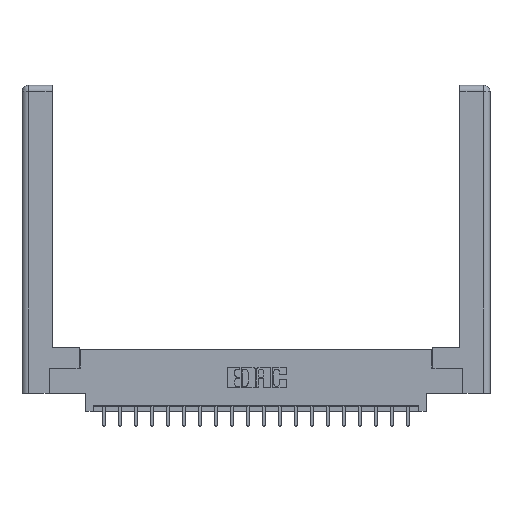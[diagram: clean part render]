
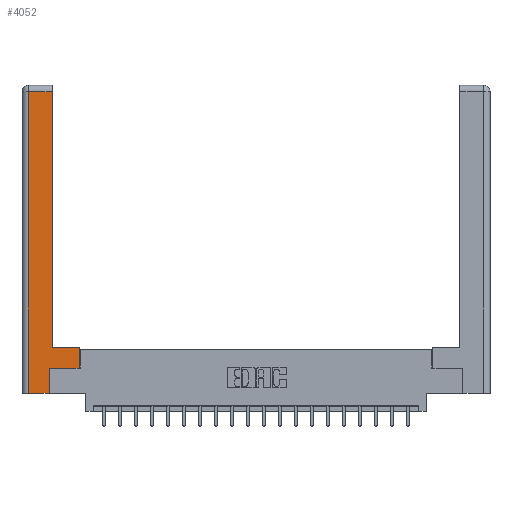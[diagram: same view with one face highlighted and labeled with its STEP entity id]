
A CAD part, top view. The second image highlights one B-rep face of the part: STEP entity #4052.
In plain terms, the highlighted planar face has unit normal (0, 0, 1).
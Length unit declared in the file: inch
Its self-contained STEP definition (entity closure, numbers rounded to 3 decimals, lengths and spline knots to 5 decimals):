
#280 = CARTESIAN_POINT ( 'NONE',  ( 0.0615, 2.94, 0. ) ) ;
#493 = DIRECTION ( 'NONE',  ( 0., 1., 0. ) ) ;
#670 = VECTOR ( 'NONE', #4784, 39.37008 ) ;
#1432 = LINE ( 'NONE', #21107, #670 ) ;
#3005 = ORIENTED_EDGE ( 'NONE', *, *, #5971, .T. ) ;
#3020 = EDGE_LOOP ( 'NONE', ( #16527, #5303, #6921, #6125, #13822, #3005, #13049, #17328 ) ) ;
#3183 = CARTESIAN_POINT ( 'NONE',  ( 0., 0., 0. ) ) ;
#4052 = ADVANCED_FACE ( 'NONE', ( #15620 ), #19458, .F. ) ;
#4313 = VERTEX_POINT ( 'NONE', #19497 ) ;
#4544 = CARTESIAN_POINT ( 'NONE',  ( 0.0615, 2.94, 0. ) ) ;
#4565 = LINE ( 'NONE', #11743, #13985 ) ;
#4569 = VERTEX_POINT ( 'NONE', #10533 ) ;
#4713 = CARTESIAN_POINT ( 'NONE',  ( 0.565, 0.245, 0. ) ) ;
#4784 = DIRECTION ( 'NONE',  ( 0., -1., 0. ) ) ;
#5303 = ORIENTED_EDGE ( 'NONE', *, *, #8015, .T. ) ;
#5707 = EDGE_CURVE ( 'NONE', #9108, #13823, #11936, .T. ) ;
#5791 = DIRECTION ( 'NONE',  ( 0., 0., -1. ) ) ;
#5861 = DIRECTION ( 'NONE',  ( -1., 0., 0. ) ) ;
#5921 = LINE ( 'NONE', #16191, #7468 ) ;
#5971 = EDGE_CURVE ( 'NONE', #13823, #10872, #4565, .T. ) ;
#6061 = CARTESIAN_POINT ( 'NONE',  ( 0.265, 0.245, 0. ) ) ;
#6125 = ORIENTED_EDGE ( 'NONE', *, *, #9671, .T. ) ;
#6391 = DIRECTION ( 'NONE',  ( 0., 1., 0. ) ) ;
#6852 = VECTOR ( 'NONE', #7717, 39.37008 ) ;
#6921 = ORIENTED_EDGE ( 'NONE', *, *, #10904, .T. ) ;
#7195 = CARTESIAN_POINT ( 'NONE',  ( 0.265, 0., 0. ) ) ;
#7468 = VECTOR ( 'NONE', #6391, 39.37008 ) ;
#7717 = DIRECTION ( 'NONE',  ( 1., 0., 0. ) ) ;
#8015 = EDGE_CURVE ( 'NONE', #4569, #14010, #19679, .T. ) ;
#9108 = VERTEX_POINT ( 'NONE', #7195 ) ;
#9671 = EDGE_CURVE ( 'NONE', #19470, #9108, #20620, .T. ) ;
#10533 = CARTESIAN_POINT ( 'NONE',  ( 0.295, 2.94, 0. ) ) ;
#10726 = EDGE_CURVE ( 'NONE', #10872, #4313, #17302, .T. ) ;
#10872 = VERTEX_POINT ( 'NONE', #4713 ) ;
#10904 = EDGE_CURVE ( 'NONE', #14010, #19470, #1432, .T. ) ;
#11191 = AXIS2_PLACEMENT_3D ( 'NONE', #3183, #5791, #5861 ) ;
#11202 = EDGE_CURVE ( 'NONE', #4313, #19335, #16265, .T. ) ;
#11743 = CARTESIAN_POINT ( 'NONE',  ( 0.565, 0.245, 0. ) ) ;
#11847 = CARTESIAN_POINT ( 'NONE',  ( 0.565, 0.45, 0. ) ) ;
#11936 = LINE ( 'NONE', #13193, #20637 ) ;
#11952 = DIRECTION ( 'NONE',  ( 1., 0., 0. ) ) ;
#12536 = VECTOR ( 'NONE', #16879, 39.37008 ) ;
#12959 = VECTOR ( 'NONE', #493, 39.37008 ) ;
#13049 = ORIENTED_EDGE ( 'NONE', *, *, #10726, .T. ) ;
#13193 = CARTESIAN_POINT ( 'NONE',  ( 0.265, 0.245, 0. ) ) ;
#13339 = DIRECTION ( 'NONE',  ( 0., 1., 0. ) ) ;
#13484 = CARTESIAN_POINT ( 'NONE',  ( 0.0615, 0., 0. ) ) ;
#13822 = ORIENTED_EDGE ( 'NONE', *, *, #5707, .T. ) ;
#13823 = VERTEX_POINT ( 'NONE', #6061 ) ;
#13985 = VECTOR ( 'NONE', #11952, 39.37008 ) ;
#14010 = VERTEX_POINT ( 'NONE', #4544 ) ;
#15620 = FACE_OUTER_BOUND ( 'NONE', #3020, .T. ) ;
#16191 = CARTESIAN_POINT ( 'NONE',  ( 0.295, 3., 0. ) ) ;
#16265 = LINE ( 'NONE', #17943, #20318 ) ;
#16527 = ORIENTED_EDGE ( 'NONE', *, *, #18765, .T. ) ;
#16879 = DIRECTION ( 'NONE',  ( -1., 0., 0. ) ) ;
#17302 = LINE ( 'NONE', #11847, #12959 ) ;
#17328 = ORIENTED_EDGE ( 'NONE', *, *, #11202, .T. ) ;
#17943 = CARTESIAN_POINT ( 'NONE',  ( 0.295, 0.45, 0. ) ) ;
#18765 = EDGE_CURVE ( 'NONE', #19335, #4569, #5921, .T. ) ;
#19335 = VERTEX_POINT ( 'NONE', #19910 ) ;
#19361 = CARTESIAN_POINT ( 'NONE',  ( 0.265, 0., 0. ) ) ;
#19458 = PLANE ( 'NONE',  #11191 ) ;
#19470 = VERTEX_POINT ( 'NONE', #13484 ) ;
#19497 = CARTESIAN_POINT ( 'NONE',  ( 0.565, 0.45, 0. ) ) ;
#19508 = DIRECTION ( 'NONE',  ( -1., 0., 0. ) ) ;
#19679 = LINE ( 'NONE', #280, #12536 ) ;
#19910 = CARTESIAN_POINT ( 'NONE',  ( 0.295, 0.45, 0. ) ) ;
#20318 = VECTOR ( 'NONE', #19508, 39.37008 ) ;
#20620 = LINE ( 'NONE', #19361, #6852 ) ;
#20637 = VECTOR ( 'NONE', #13339, 39.37008 ) ;
#21107 = CARTESIAN_POINT ( 'NONE',  ( 0.0615, 0., 0. ) ) ;
